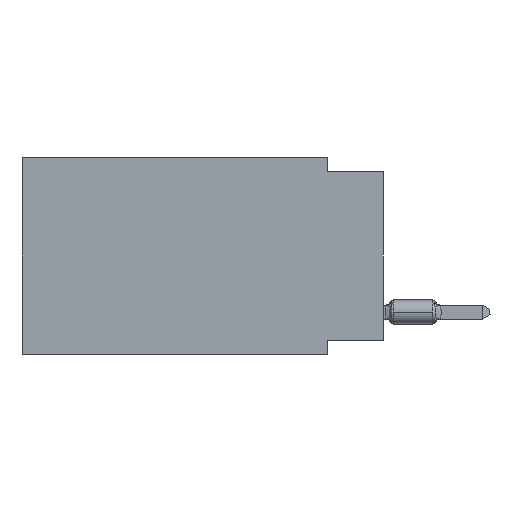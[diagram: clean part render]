
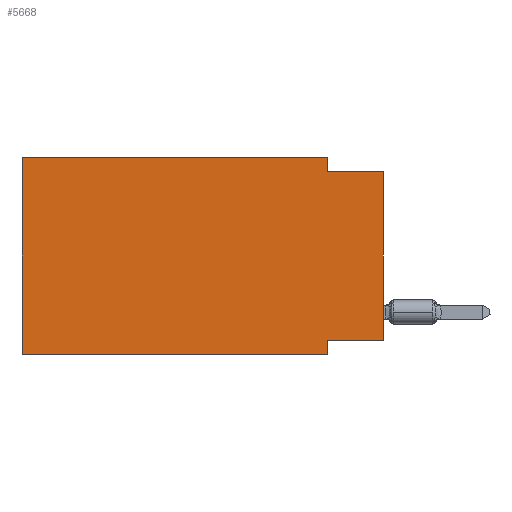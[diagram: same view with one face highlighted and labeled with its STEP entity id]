
A CAD part, left-side view. The second image highlights one B-rep face of the part: STEP entity #5668.
In plain terms, the highlighted planar face has unit normal (-1, 0, 0).
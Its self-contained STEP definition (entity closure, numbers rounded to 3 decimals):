
#512 = DIRECTION ( 'NONE',  ( 0., 0., 1. ) ) ;
#818 = EDGE_CURVE ( 'NONE', #1567, #72004, #35722, .T. ) ;
#1567 = VERTEX_POINT ( 'NONE', #81633 ) ;
#1656 = CARTESIAN_POINT ( 'NONE',  ( 0., 16.383, 0. ) ) ;
#2532 = DIRECTION ( 'NONE',  ( 0., -1., 0. ) ) ;
#3802 = EDGE_CURVE ( 'NONE', #43586, #89324, #57565, .T. ) ;
#5668 = ADVANCED_FACE ( 'NONE', ( #7195 ), #20931, .F. ) ;
#5937 = LINE ( 'NONE', #60464, #82430 ) ;
#7195 = FACE_OUTER_BOUND ( 'NONE', #36957, .T. ) ;
#7741 = CARTESIAN_POINT ( 'NONE',  ( 0., 2.54, -0.635 ) ) ;
#7758 = ORIENTED_EDGE ( 'NONE', *, *, #83320, .F. ) ;
#8778 = VERTEX_POINT ( 'NONE', #89000 ) ;
#10545 = VECTOR ( 'NONE', #78699, 1000. ) ;
#10839 = CARTESIAN_POINT ( 'NONE',  ( 0., 16.383, 0. ) ) ;
#12040 = ORIENTED_EDGE ( 'NONE', *, *, #62811, .F. ) ;
#12805 = DIRECTION ( 'NONE',  ( 0., 1., 0. ) ) ;
#13325 = ORIENTED_EDGE ( 'NONE', *, *, #89218, .T. ) ;
#14438 = EDGE_CURVE ( 'NONE', #8778, #43586, #5937, .T. ) ;
#15508 = CARTESIAN_POINT ( 'NONE',  ( 0., 16.383, 0. ) ) ;
#17889 = VECTOR ( 'NONE', #46013, 1000. ) ;
#18627 = AXIS2_PLACEMENT_3D ( 'NONE', #1656, #83669, #63065 ) ;
#18956 = CARTESIAN_POINT ( 'NONE',  ( 0., 16.383, -8.89 ) ) ;
#20267 = ORIENTED_EDGE ( 'NONE', *, *, #86132, .F. ) ;
#20615 = CARTESIAN_POINT ( 'NONE',  ( 0., 2.54, 0. ) ) ;
#20931 = PLANE ( 'NONE',  #18627 ) ;
#23063 = ORIENTED_EDGE ( 'NONE', *, *, #818, .F. ) ;
#24521 = VERTEX_POINT ( 'NONE', #84725 ) ;
#28834 = EDGE_CURVE ( 'NONE', #73440, #89324, #67056, .T. ) ;
#31160 = CARTESIAN_POINT ( 'NONE',  ( 0., 2.54, -8.89 ) ) ;
#31852 = VECTOR ( 'NONE', #37855, 1000. ) ;
#31990 = CARTESIAN_POINT ( 'NONE',  ( 0., 16.383, -8.89 ) ) ;
#32358 = LINE ( 'NONE', #10839, #57567 ) ;
#35662 = CARTESIAN_POINT ( 'NONE',  ( 0., 2.54, -8.255 ) ) ;
#35722 = LINE ( 'NONE', #20615, #44601 ) ;
#36899 = CARTESIAN_POINT ( 'NONE',  ( 0., 0., -0.635 ) ) ;
#36957 = EDGE_LOOP ( 'NONE', ( #13325, #20267, #23063, #12040, #7758, #77113, #37625, #84343 ) ) ;
#37625 = ORIENTED_EDGE ( 'NONE', *, *, #3802, .F. ) ;
#37855 = DIRECTION ( 'NONE',  ( 0., 0., -1. ) ) ;
#40501 = CARTESIAN_POINT ( 'NONE',  ( 0., 0., -0.635 ) ) ;
#42652 = LINE ( 'NONE', #77001, #66896 ) ;
#43586 = VERTEX_POINT ( 'NONE', #35662 ) ;
#44601 = VECTOR ( 'NONE', #61862, 1000. ) ;
#45608 = LINE ( 'NONE', #15508, #10545 ) ;
#46013 = DIRECTION ( 'NONE',  ( 0., -1., 0. ) ) ;
#47465 = DIRECTION ( 'NONE',  ( 0., 0., 1. ) ) ;
#57565 = LINE ( 'NONE', #71752, #31852 ) ;
#57567 = VECTOR ( 'NONE', #47465, 1000. ) ;
#60464 = CARTESIAN_POINT ( 'NONE',  ( 0., 0., -8.255 ) ) ;
#60606 = VERTEX_POINT ( 'NONE', #40501 ) ;
#61862 = DIRECTION ( 'NONE',  ( 0., 0., -1. ) ) ;
#62811 = EDGE_CURVE ( 'NONE', #24521, #1567, #45608, .T. ) ;
#63065 = DIRECTION ( 'NONE',  ( 0., 0., -1. ) ) ;
#66896 = VECTOR ( 'NONE', #512, 1000. ) ;
#67056 = LINE ( 'NONE', #18956, #17889 ) ;
#69656 = VECTOR ( 'NONE', #2532, 1000. ) ;
#71752 = CARTESIAN_POINT ( 'NONE',  ( 0., 2.54, -8.89 ) ) ;
#72004 = VERTEX_POINT ( 'NONE', #7741 ) ;
#73063 = LINE ( 'NONE', #36899, #69656 ) ;
#73440 = VERTEX_POINT ( 'NONE', #31990 ) ;
#77001 = CARTESIAN_POINT ( 'NONE',  ( 0., 0., 0. ) ) ;
#77113 = ORIENTED_EDGE ( 'NONE', *, *, #28834, .T. ) ;
#78699 = DIRECTION ( 'NONE',  ( 0., -1., 0. ) ) ;
#81633 = CARTESIAN_POINT ( 'NONE',  ( 0., 2.54, 0. ) ) ;
#82430 = VECTOR ( 'NONE', #12805, 1000. ) ;
#83320 = EDGE_CURVE ( 'NONE', #73440, #24521, #32358, .T. ) ;
#83669 = DIRECTION ( 'NONE',  ( 1., 0., 0. ) ) ;
#84343 = ORIENTED_EDGE ( 'NONE', *, *, #14438, .F. ) ;
#84725 = CARTESIAN_POINT ( 'NONE',  ( 0., 16.383, 0. ) ) ;
#86132 = EDGE_CURVE ( 'NONE', #72004, #60606, #73063, .T. ) ;
#89000 = CARTESIAN_POINT ( 'NONE',  ( 0., 0., -8.255 ) ) ;
#89218 = EDGE_CURVE ( 'NONE', #8778, #60606, #42652, .T. ) ;
#89324 = VERTEX_POINT ( 'NONE', #31160 ) ;
